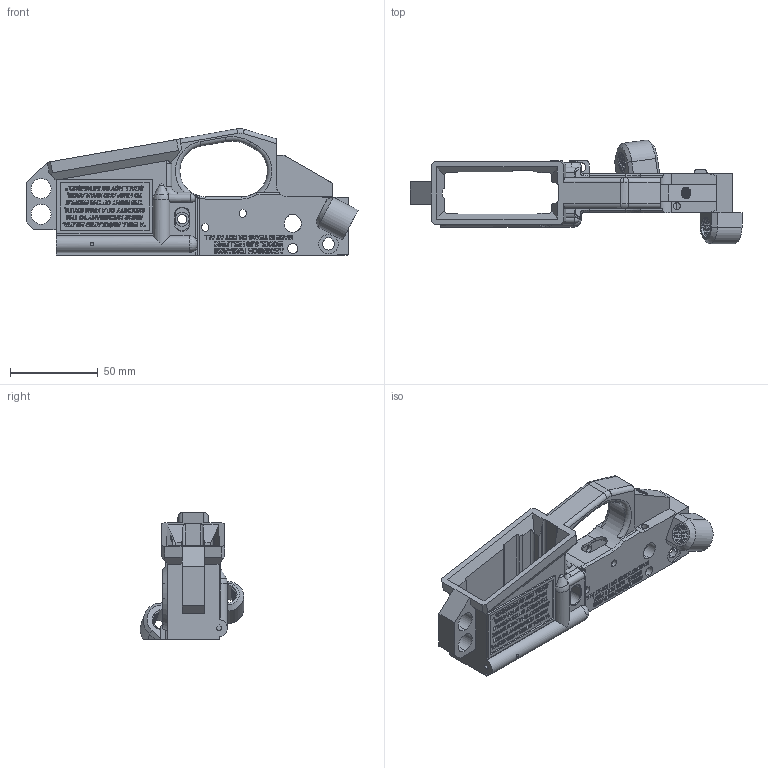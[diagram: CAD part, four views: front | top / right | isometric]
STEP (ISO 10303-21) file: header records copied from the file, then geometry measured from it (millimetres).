
FILE_DESCRIPTION (( 'STEP AP203' ), '1' );
FILE_NAME ('AF-HF-LR-PRT-FA-NS-001-STEP.STEP', '2020-12-05T02:21:33', ( '' ), ( '' ), 'SwSTEP 2.0', 'SolidWorks 2018', '' );
FILE_SCHEMA (( 'CONFIG_CONTROL_DESIGN' ));
Length unit declared in the file: inch
Products named in the file (1): AF-HF-LR-PRT-FA-NS-001-STEP
Bounding box: 189.54 x 59.15 x 72.31 mm (x, y, z)
Volume: 98038.5 mm3; surface area: 58618 mm2
Topology: 1 solids, 1 shells, 3153 faces, 8639 edges, 5722 vertices
Faces by surface type: plane 2101, bspline 759, cylinder 248, torus 22, cone 19, sphere 4
Entity records: 180143 total; most frequent: CARTESIAN_POINT 106243, ORIENTED_EDGE 17266, DIRECTION 11886, EDGE_CURVE 8633, VECTOR 6322, LINE 6322, VERTEX_POINT 5721, EDGE_LOOP 3442
